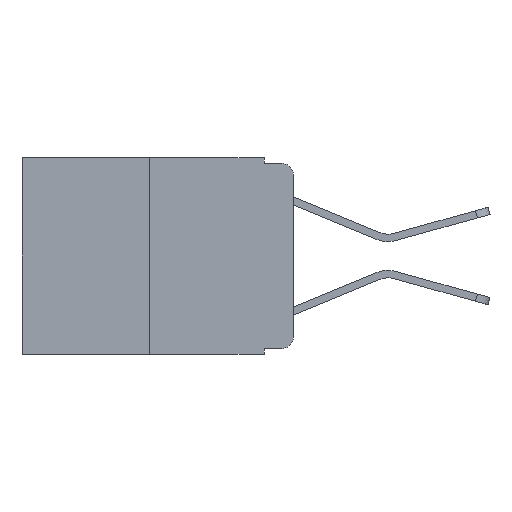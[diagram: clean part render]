
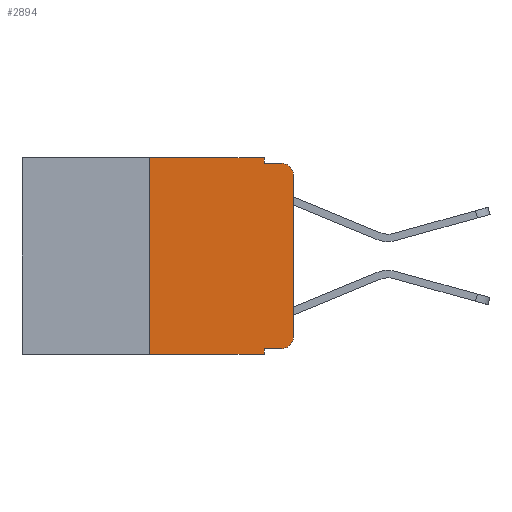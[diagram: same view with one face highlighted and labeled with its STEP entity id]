
A CAD part, left-side view. The second image highlights one B-rep face of the part: STEP entity #2894.
In plain terms, the highlighted planar face has unit normal (-1, 0, 0).
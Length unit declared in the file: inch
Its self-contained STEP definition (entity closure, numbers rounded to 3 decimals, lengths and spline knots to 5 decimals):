
#289 = VECTOR ( 'NONE', #8058, 39.37008 ) ;
#484 = ORIENTED_EDGE ( 'NONE', *, *, #1643, .F. ) ;
#493 = EDGE_CURVE ( 'NONE', #9108, #13961, #9986, .T. ) ;
#619 = CARTESIAN_POINT ( 'NONE',  ( 0., 0.051, -0.343 ) ) ;
#954 = CARTESIAN_POINT ( 'NONE',  ( 0., 0.473, 0. ) ) ;
#973 = DIRECTION ( 'NONE',  ( 0., -1., 0. ) ) ;
#1158 = ORIENTED_EDGE ( 'NONE', *, *, #3008, .F. ) ;
#1203 = CARTESIAN_POINT ( 'NONE',  ( 0., 0.25, -0.343 ) ) ;
#1232 = LINE ( 'NONE', #5603, #3339 ) ;
#1426 = ORIENTED_EDGE ( 'NONE', *, *, #10450, .F. ) ;
#1643 = EDGE_CURVE ( 'NONE', #3688, #13961, #6089, .T. ) ;
#1676 = VECTOR ( 'NONE', #2625, 39.37008 ) ;
#1721 = VERTEX_POINT ( 'NONE', #619 ) ;
#1725 = CARTESIAN_POINT ( 'NONE',  ( 0., 0.02, -0.03 ) ) ;
#2240 = PLANE ( 'NONE',  #9256 ) ;
#2264 = LINE ( 'NONE', #4415, #8974 ) ;
#2625 = DIRECTION ( 'NONE',  ( 0., 0., -1. ) ) ;
#2649 = ORIENTED_EDGE ( 'NONE', *, *, #7985, .T. ) ;
#2864 = DIRECTION ( 'NONE',  ( 0., -1., 0. ) ) ;
#2894 = ADVANCED_FACE ( 'NONE', ( #7765 ), #2240, .F. ) ;
#3008 = EDGE_CURVE ( 'NONE', #8055, #3819, #13319, .T. ) ;
#3009 = VECTOR ( 'NONE', #7836, 39.37008 ) ;
#3122 = LINE ( 'NONE', #7499, #8273 ) ;
#3140 = AXIS2_PLACEMENT_3D ( 'NONE', #1725, #12700, #13722 ) ;
#3339 = VECTOR ( 'NONE', #7977, 39.37008 ) ;
#3456 = CARTESIAN_POINT ( 'NONE',  ( 0., 0.051, -0.01 ) ) ;
#3688 = VERTEX_POINT ( 'NONE', #12104 ) ;
#3694 = CARTESIAN_POINT ( 'NONE',  ( 0., 0.051, 0. ) ) ;
#3819 = VERTEX_POINT ( 'NONE', #3694 ) ;
#4165 = AXIS2_PLACEMENT_3D ( 'NONE', #4786, #4930, #9281 ) ;
#4415 = CARTESIAN_POINT ( 'NONE',  ( 0., 0.051, -0.333 ) ) ;
#4467 = DIRECTION ( 'NONE',  ( 1., 0., 0. ) ) ;
#4716 = EDGE_CURVE ( 'NONE', #9298, #1721, #7163, .T. ) ;
#4786 = CARTESIAN_POINT ( 'NONE',  ( 0., 0.02, -0.313 ) ) ;
#4930 = DIRECTION ( 'NONE',  ( -1., 0., 0. ) ) ;
#5114 = ORIENTED_EDGE ( 'NONE', *, *, #493, .T. ) ;
#5539 = DIRECTION ( 'NONE',  ( 0., 0., -1. ) ) ;
#5593 = CARTESIAN_POINT ( 'NONE',  ( 0., 0.051, -0.333 ) ) ;
#5603 = CARTESIAN_POINT ( 'NONE',  ( 0., 0.25, 0. ) ) ;
#5686 = CARTESIAN_POINT ( 'NONE',  ( 0., 0.25, 0. ) ) ;
#5698 = LINE ( 'NONE', #7934, #1676 ) ;
#5896 = LINE ( 'NONE', #11295, #289 ) ;
#6033 = ORIENTED_EDGE ( 'NONE', *, *, #4716, .T. ) ;
#6089 = LINE ( 'NONE', #3456, #3009 ) ;
#6776 = DIRECTION ( 'NONE',  ( 0., -1., 0. ) ) ;
#6981 = CARTESIAN_POINT ( 'NONE',  ( 0., 0.02, -0.01 ) ) ;
#7163 = LINE ( 'NONE', #11406, #12528 ) ;
#7433 = CARTESIAN_POINT ( 'NONE',  ( 0., 0., -0.313 ) ) ;
#7499 = CARTESIAN_POINT ( 'NONE',  ( 0., 0., 0. ) ) ;
#7765 = FACE_OUTER_BOUND ( 'NONE', #10981, .T. ) ;
#7836 = DIRECTION ( 'NONE',  ( 0., -1., 0. ) ) ;
#7934 = CARTESIAN_POINT ( 'NONE',  ( 0., 0.051, 0. ) ) ;
#7977 = DIRECTION ( 'NONE',  ( 0., 0., 1. ) ) ;
#7985 = EDGE_CURVE ( 'NONE', #13087, #9108, #3122, .T. ) ;
#8055 = VERTEX_POINT ( 'NONE', #5686 ) ;
#8058 = DIRECTION ( 'NONE',  ( 0., 0., -1. ) ) ;
#8273 = VECTOR ( 'NONE', #10347, 39.37008 ) ;
#8620 = ORIENTED_EDGE ( 'NONE', *, *, #9755, .T. ) ;
#8974 = VECTOR ( 'NONE', #973, 39.37008 ) ;
#9019 = CARTESIAN_POINT ( 'NONE',  ( 0., 0.02, -0.333 ) ) ;
#9108 = VERTEX_POINT ( 'NONE', #13241 ) ;
#9256 = AXIS2_PLACEMENT_3D ( 'NONE', #954, #4467, #5539 ) ;
#9281 = DIRECTION ( 'NONE',  ( 0., 0., -1. ) ) ;
#9298 = VERTEX_POINT ( 'NONE', #1203 ) ;
#9394 = ORIENTED_EDGE ( 'NONE', *, *, #13972, .F. ) ;
#9502 = EDGE_CURVE ( 'NONE', #10920, #13087, #10323, .T. ) ;
#9755 = EDGE_CURVE ( 'NONE', #10797, #10920, #2264, .T. ) ;
#9883 = EDGE_CURVE ( 'NONE', #10797, #1721, #5698, .T. ) ;
#9986 = CIRCLE ( 'NONE', #3140, 0.02 ) ;
#10323 = CIRCLE ( 'NONE', #4165, 0.02 ) ;
#10347 = DIRECTION ( 'NONE',  ( 0., 0., 1. ) ) ;
#10450 = EDGE_CURVE ( 'NONE', #3819, #3688, #5896, .T. ) ;
#10797 = VERTEX_POINT ( 'NONE', #5593 ) ;
#10920 = VERTEX_POINT ( 'NONE', #9019 ) ;
#10981 = EDGE_LOOP ( 'NONE', ( #2649, #5114, #484, #1426, #1158, #9394, #6033, #13911, #8620, #13371 ) ) ;
#11295 = CARTESIAN_POINT ( 'NONE',  ( 0., 0.051, 0. ) ) ;
#11406 = CARTESIAN_POINT ( 'NONE',  ( 0., 0.473, -0.343 ) ) ;
#12104 = CARTESIAN_POINT ( 'NONE',  ( 0., 0.051, -0.01 ) ) ;
#12226 = CARTESIAN_POINT ( 'NONE',  ( 0., 0.473, 0. ) ) ;
#12528 = VECTOR ( 'NONE', #2864, 39.37008 ) ;
#12700 = DIRECTION ( 'NONE',  ( -1., 0., 0. ) ) ;
#12780 = VECTOR ( 'NONE', #6776, 39.37008 ) ;
#13087 = VERTEX_POINT ( 'NONE', #7433 ) ;
#13241 = CARTESIAN_POINT ( 'NONE',  ( 0., 0., -0.03 ) ) ;
#13319 = LINE ( 'NONE', #12226, #12780 ) ;
#13371 = ORIENTED_EDGE ( 'NONE', *, *, #9502, .T. ) ;
#13722 = DIRECTION ( 'NONE',  ( 0., 0., -1. ) ) ;
#13911 = ORIENTED_EDGE ( 'NONE', *, *, #9883, .F. ) ;
#13961 = VERTEX_POINT ( 'NONE', #6981 ) ;
#13972 = EDGE_CURVE ( 'NONE', #9298, #8055, #1232, .T. ) ;
